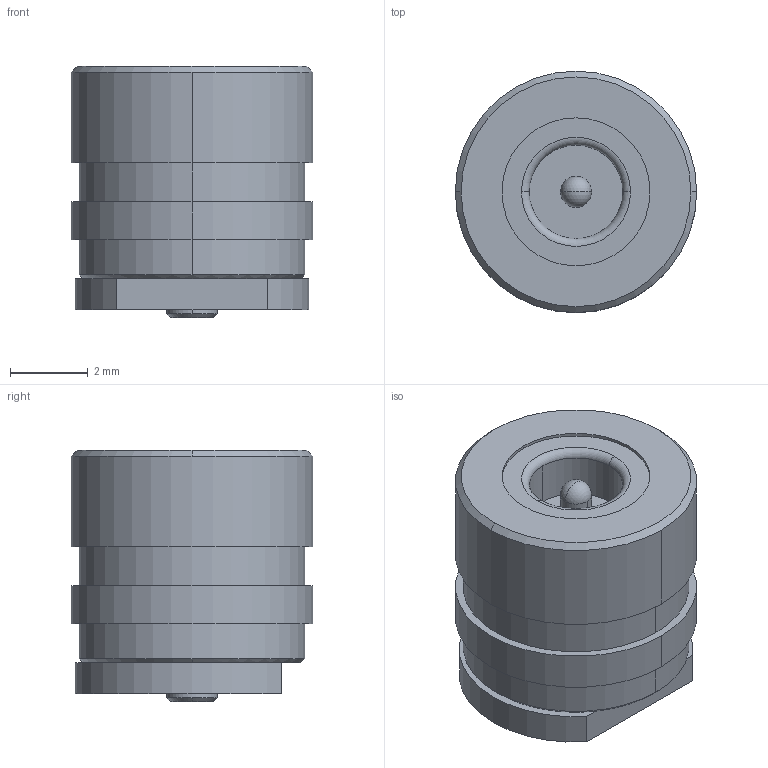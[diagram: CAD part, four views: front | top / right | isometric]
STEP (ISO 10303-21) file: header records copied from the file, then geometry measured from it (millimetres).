
FILE_DESCRIPTION (( 'STEP AP203' ), '1' );
FILE_NAME ('686-B02C2P001B0.STEP', '2023-02-14T09:22:38', ( 'Magnum' ), ( '' ), 'SwSTEP 2.0', 'SolidWorks 2020', '' );
FILE_SCHEMA (( 'CONFIG_CONTROL_DESIGN' ));
Length unit declared in the file: millimetre
Products named in the file (1): 686-B02C2P001B0
Bounding box: 6.2 x 6.2 x 6.45 mm (x, y, z)
Volume: 164.4 mm3; surface area: 362.6 mm2
Topology: 1 solids, 5 shells, 67 faces, 153 edges, 100 vertices
Faces by surface type: cylinder 31, plane 18, torus 10, cone 6, sphere 2
Entity records: 2023 total; most frequent: DIRECTION 396, CARTESIAN_POINT 319, ORIENTED_EDGE 302, AXIS2_PLACEMENT_3D 177, EDGE_CURVE 151, CIRCLE 109, VERTEX_POINT 100, EDGE_LOOP 81
